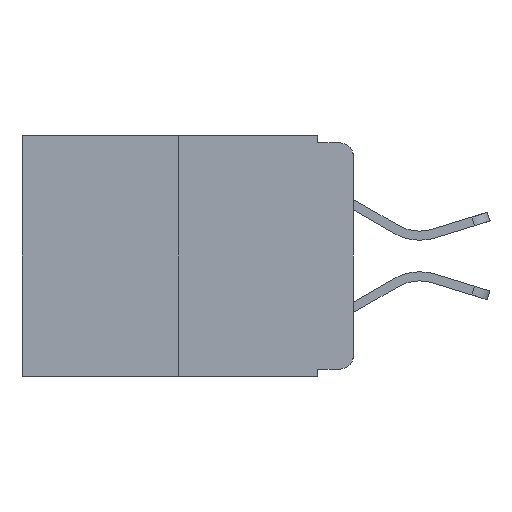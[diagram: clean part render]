
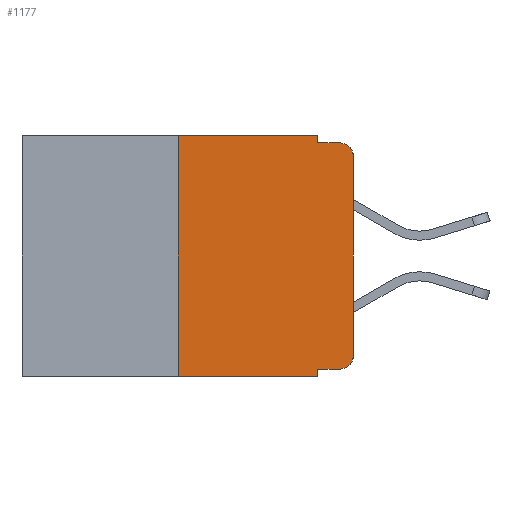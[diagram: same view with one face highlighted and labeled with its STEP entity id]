
A CAD part, left-side view. The second image highlights one B-rep face of the part: STEP entity #1177.
In plain terms, the highlighted planar face has unit normal (-1, 0, 0).
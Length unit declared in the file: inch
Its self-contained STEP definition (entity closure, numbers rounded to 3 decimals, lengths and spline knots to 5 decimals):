
#83 = ORIENTED_EDGE ( 'NONE', *, *, #3138, .F. ) ;
#211 = AXIS2_PLACEMENT_3D ( 'NONE', #8763, #7162, #10024 ) ;
#283 = VERTEX_POINT ( 'NONE', #9838 ) ;
#414 = AXIS2_PLACEMENT_3D ( 'NONE', #9597, #9504, #7026 ) ;
#838 = CARTESIAN_POINT ( 'NONE',  ( 0., 0.051, -0.333 ) ) ;
#1177 = ADVANCED_FACE ( 'NONE', ( #6176 ), #10151, .F. ) ;
#1295 = VERTEX_POINT ( 'NONE', #6610 ) ;
#1411 = LINE ( 'NONE', #9822, #7918 ) ;
#1614 = LINE ( 'NONE', #9746, #6709 ) ;
#1800 = CARTESIAN_POINT ( 'NONE',  ( 0., 0.051, -0.01 ) ) ;
#1830 = ORIENTED_EDGE ( 'NONE', *, *, #4175, .T. ) ;
#2244 = VERTEX_POINT ( 'NONE', #5902 ) ;
#2340 = VECTOR ( 'NONE', #9000, 39.37008 ) ;
#2406 = DIRECTION ( 'NONE',  ( 0., -1., 0. ) ) ;
#2447 = CARTESIAN_POINT ( 'NONE',  ( 0., 0.473, 0. ) ) ;
#2842 = DIRECTION ( 'NONE',  ( 0., 0., -1. ) ) ;
#2860 = VERTEX_POINT ( 'NONE', #10148 ) ;
#2900 = LINE ( 'NONE', #10087, #2340 ) ;
#2948 = AXIS2_PLACEMENT_3D ( 'NONE', #2447, #8742, #2842 ) ;
#3138 = EDGE_CURVE ( 'NONE', #4951, #283, #1614, .T. ) ;
#3283 = DIRECTION ( 'NONE',  ( 0., 0., 1. ) ) ;
#3529 = VERTEX_POINT ( 'NONE', #6289 ) ;
#3759 = EDGE_CURVE ( 'NONE', #1295, #4121, #9434, .T. ) ;
#4121 = VERTEX_POINT ( 'NONE', #5824 ) ;
#4175 = EDGE_CURVE ( 'NONE', #2860, #2244, #6947, .T. ) ;
#4244 = EDGE_CURVE ( 'NONE', #2244, #3529, #5599, .T. ) ;
#4270 = VERTEX_POINT ( 'NONE', #9318 ) ;
#4279 = EDGE_CURVE ( 'NONE', #9692, #3529, #2900, .T. ) ;
#4296 = EDGE_CURVE ( 'NONE', #283, #9692, #4481, .T. ) ;
#4312 = EDGE_CURVE ( 'NONE', #1295, #4951, #8555, .T. ) ;
#4334 = EDGE_CURVE ( 'NONE', #4270, #4121, #1411, .T. ) ;
#4347 = EDGE_CURVE ( 'NONE', #4270, #9902, #9739, .T. ) ;
#4481 = LINE ( 'NONE', #6951, #10368 ) ;
#4509 = EDGE_CURVE ( 'NONE', #9902, #2860, #7221, .T. ) ;
#4575 = EDGE_LOOP ( 'NONE', ( #1830, #8812, #10614, #9023, #83, #5069, #7594, #9446, #7841, #9665 ) ) ;
#4951 = VERTEX_POINT ( 'NONE', #7034 ) ;
#5069 = ORIENTED_EDGE ( 'NONE', *, *, #4312, .F. ) ;
#5599 = CIRCLE ( 'NONE', #414, 0.02 ) ;
#5824 = CARTESIAN_POINT ( 'NONE',  ( 0., 0.051, -0.343 ) ) ;
#5902 = CARTESIAN_POINT ( 'NONE',  ( 0., 0., -0.03 ) ) ;
#6176 = FACE_OUTER_BOUND ( 'NONE', #4575, .T. ) ;
#6289 = CARTESIAN_POINT ( 'NONE',  ( 0., 0.02, -0.01 ) ) ;
#6605 = DIRECTION ( 'NONE',  ( 0., -1., 0. ) ) ;
#6610 = CARTESIAN_POINT ( 'NONE',  ( 0., 0.25, -0.343 ) ) ;
#6709 = VECTOR ( 'NONE', #9677, 39.37008 ) ;
#6947 = LINE ( 'NONE', #10474, #8675 ) ;
#6951 = CARTESIAN_POINT ( 'NONE',  ( 0., 0.051, 0. ) ) ;
#7026 = DIRECTION ( 'NONE',  ( 0., 0., -1. ) ) ;
#7034 = CARTESIAN_POINT ( 'NONE',  ( 0., 0.25, 0. ) ) ;
#7162 = DIRECTION ( 'NONE',  ( -1., 0., 0. ) ) ;
#7221 = CIRCLE ( 'NONE', #211, 0.02 ) ;
#7594 = ORIENTED_EDGE ( 'NONE', *, *, #3759, .T. ) ;
#7826 = VECTOR ( 'NONE', #2406, 39.37008 ) ;
#7841 = ORIENTED_EDGE ( 'NONE', *, *, #4347, .T. ) ;
#7918 = VECTOR ( 'NONE', #8188, 39.37008 ) ;
#8188 = DIRECTION ( 'NONE',  ( 0., 0., -1. ) ) ;
#8274 = DIRECTION ( 'NONE',  ( 0., 0., -1. ) ) ;
#8555 = LINE ( 'NONE', #8858, #10160 ) ;
#8675 = VECTOR ( 'NONE', #3283, 39.37008 ) ;
#8742 = DIRECTION ( 'NONE',  ( 1., 0., 0. ) ) ;
#8763 = CARTESIAN_POINT ( 'NONE',  ( 0., 0.02, -0.313 ) ) ;
#8812 = ORIENTED_EDGE ( 'NONE', *, *, #4244, .T. ) ;
#8858 = CARTESIAN_POINT ( 'NONE',  ( 0., 0.25, 0. ) ) ;
#9000 = DIRECTION ( 'NONE',  ( 0., -1., 0. ) ) ;
#9023 = ORIENTED_EDGE ( 'NONE', *, *, #4296, .F. ) ;
#9318 = CARTESIAN_POINT ( 'NONE',  ( 0., 0.051, -0.333 ) ) ;
#9434 = LINE ( 'NONE', #9716, #7826 ) ;
#9446 = ORIENTED_EDGE ( 'NONE', *, *, #4334, .F. ) ;
#9504 = DIRECTION ( 'NONE',  ( -1., 0., 0. ) ) ;
#9524 = VECTOR ( 'NONE', #6605, 39.37008 ) ;
#9597 = CARTESIAN_POINT ( 'NONE',  ( 0., 0.02, -0.03 ) ) ;
#9665 = ORIENTED_EDGE ( 'NONE', *, *, #4509, .T. ) ;
#9677 = DIRECTION ( 'NONE',  ( 0., -1., 0. ) ) ;
#9692 = VERTEX_POINT ( 'NONE', #1800 ) ;
#9716 = CARTESIAN_POINT ( 'NONE',  ( 0., 0.473, -0.343 ) ) ;
#9739 = LINE ( 'NONE', #838, #9524 ) ;
#9746 = CARTESIAN_POINT ( 'NONE',  ( 0., 0.473, 0. ) ) ;
#9785 = DIRECTION ( 'NONE',  ( 0., 0., 1. ) ) ;
#9822 = CARTESIAN_POINT ( 'NONE',  ( 0., 0.051, 0. ) ) ;
#9838 = CARTESIAN_POINT ( 'NONE',  ( 0., 0.051, 0. ) ) ;
#9902 = VERTEX_POINT ( 'NONE', #10735 ) ;
#10024 = DIRECTION ( 'NONE',  ( 0., 0., -1. ) ) ;
#10087 = CARTESIAN_POINT ( 'NONE',  ( 0., 0.051, -0.01 ) ) ;
#10148 = CARTESIAN_POINT ( 'NONE',  ( 0., 0., -0.313 ) ) ;
#10151 = PLANE ( 'NONE',  #2948 ) ;
#10160 = VECTOR ( 'NONE', #9785, 39.37008 ) ;
#10368 = VECTOR ( 'NONE', #8274, 39.37008 ) ;
#10474 = CARTESIAN_POINT ( 'NONE',  ( 0., 0., 0. ) ) ;
#10614 = ORIENTED_EDGE ( 'NONE', *, *, #4279, .F. ) ;
#10735 = CARTESIAN_POINT ( 'NONE',  ( 0., 0.02, -0.333 ) ) ;
